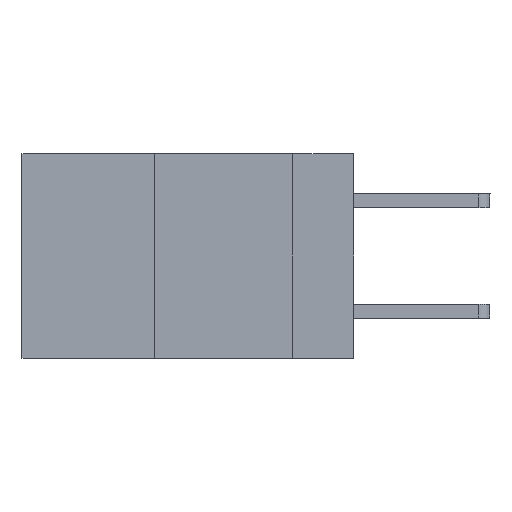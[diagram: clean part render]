
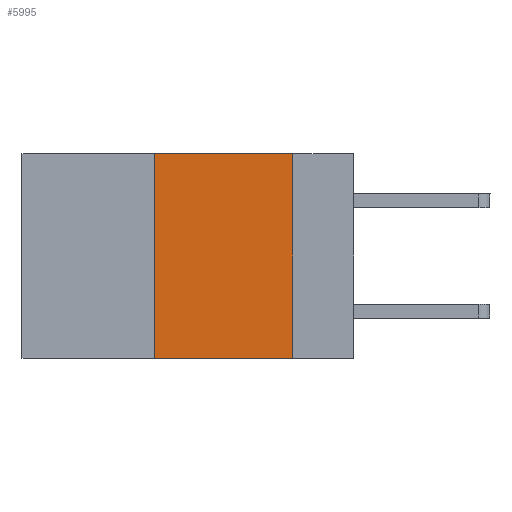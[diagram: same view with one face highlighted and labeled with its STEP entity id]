
A CAD part, left-side view. The second image highlights one B-rep face of the part: STEP entity #5995.
In plain terms, the highlighted planar face has unit normal (-1, 0, 0).
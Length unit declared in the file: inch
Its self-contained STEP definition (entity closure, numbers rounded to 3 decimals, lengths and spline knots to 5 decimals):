
#568 = ORIENTED_EDGE ( 'NONE', *, *, #2314, .F. ) ;
#590 = VERTEX_POINT ( 'NONE', #1688 ) ;
#786 = LINE ( 'NONE', #7239, #3349 ) ;
#1502 = CARTESIAN_POINT ( 'NONE',  ( 0., 0.36, 0. ) ) ;
#1688 = CARTESIAN_POINT ( 'NONE',  ( 0., 0.36, -0.37 ) ) ;
#1937 = VECTOR ( 'NONE', #5561, 39.37008 ) ;
#2287 = VERTEX_POINT ( 'NONE', #11876 ) ;
#2314 = EDGE_CURVE ( 'NONE', #10610, #2287, #786, .T. ) ;
#2497 = DIRECTION ( 'NONE',  ( 0., 0., 1. ) ) ;
#2638 = DIRECTION ( 'NONE',  ( 0., 0., -1. ) ) ;
#2686 = LINE ( 'NONE', #1502, #4521 ) ;
#2792 = CARTESIAN_POINT ( 'NONE',  ( 0., 0.6, -0.37 ) ) ;
#3349 = VECTOR ( 'NONE', #8181, 39.37008 ) ;
#3696 = AXIS2_PLACEMENT_3D ( 'NONE', #5300, #8069, #2638 ) ;
#3975 = CARTESIAN_POINT ( 'NONE',  ( 0., 0.6, 0. ) ) ;
#4521 = VECTOR ( 'NONE', #2497, 39.37008 ) ;
#5300 = CARTESIAN_POINT ( 'NONE',  ( 0., 0.6, 0. ) ) ;
#5328 = EDGE_CURVE ( 'NONE', #590, #9241, #2686, .T. ) ;
#5561 = DIRECTION ( 'NONE',  ( 0., -1., 0. ) ) ;
#5802 = EDGE_LOOP ( 'NONE', ( #568, #10506, #10792, #8578 ) ) ;
#5995 = ADVANCED_FACE ( 'NONE', ( #6431 ), #11768, .F. ) ;
#6431 = FACE_OUTER_BOUND ( 'NONE', #5802, .T. ) ;
#6537 = VECTOR ( 'NONE', #10402, 39.37008 ) ;
#7239 = CARTESIAN_POINT ( 'NONE',  ( 0., 0.11, 0. ) ) ;
#7771 = CARTESIAN_POINT ( 'NONE',  ( 0., 0.36, 0. ) ) ;
#8069 = DIRECTION ( 'NONE',  ( 1., 0., 0. ) ) ;
#8181 = DIRECTION ( 'NONE',  ( 0., 0., -1. ) ) ;
#8449 = LINE ( 'NONE', #3975, #6537 ) ;
#8578 = ORIENTED_EDGE ( 'NONE', *, *, #10294, .T. ) ;
#9241 = VERTEX_POINT ( 'NONE', #7771 ) ;
#9252 = LINE ( 'NONE', #2792, #1937 ) ;
#10294 = EDGE_CURVE ( 'NONE', #590, #2287, #9252, .T. ) ;
#10386 = CARTESIAN_POINT ( 'NONE',  ( 0., 0.11, 0. ) ) ;
#10402 = DIRECTION ( 'NONE',  ( 0., -1., 0. ) ) ;
#10506 = ORIENTED_EDGE ( 'NONE', *, *, #11951, .F. ) ;
#10610 = VERTEX_POINT ( 'NONE', #10386 ) ;
#10792 = ORIENTED_EDGE ( 'NONE', *, *, #5328, .F. ) ;
#11768 = PLANE ( 'NONE',  #3696 ) ;
#11876 = CARTESIAN_POINT ( 'NONE',  ( 0., 0.11, -0.37 ) ) ;
#11951 = EDGE_CURVE ( 'NONE', #9241, #10610, #8449, .T. ) ;
